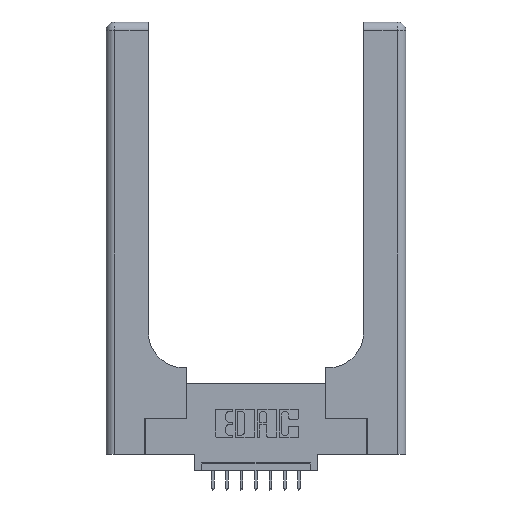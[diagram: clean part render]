
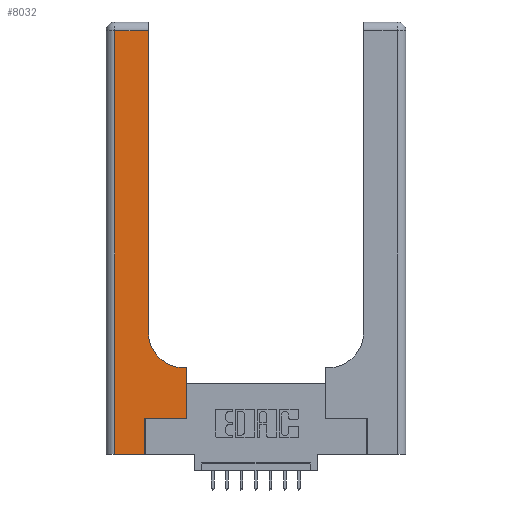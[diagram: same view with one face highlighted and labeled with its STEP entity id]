
A CAD part, top view. The second image highlights one B-rep face of the part: STEP entity #8032.
In plain terms, the highlighted planar face has unit normal (0, 0, 1).
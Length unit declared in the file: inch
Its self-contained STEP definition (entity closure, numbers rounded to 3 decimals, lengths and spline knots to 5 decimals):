
#13 = CARTESIAN_POINT ( 'NONE',  ( 0.5415, 0.85, 0.37 ) ) ;
#379 = EDGE_CURVE ( 'NONE', #5066, #6517, #4781, .T. ) ;
#677 = VERTEX_POINT ( 'NONE', #11821 ) ;
#979 = VERTEX_POINT ( 'NONE', #9960 ) ;
#1212 = DIRECTION ( 'NONE',  ( -1., 0., 0. ) ) ;
#1275 = CARTESIAN_POINT ( 'NONE',  ( 0.5585, 0.6, 0.37 ) ) ;
#1513 = EDGE_CURVE ( 'NONE', #6517, #6778, #9092, .T. ) ;
#1852 = ORIENTED_EDGE ( 'NONE', *, *, #12530, .T. ) ;
#1937 = ORIENTED_EDGE ( 'NONE', *, *, #12437, .T. ) ;
#2264 = CARTESIAN_POINT ( 'NONE',  ( 0.2915, 2.94, 0.37 ) ) ;
#2290 = CARTESIAN_POINT ( 'NONE',  ( 0., 0., 0.37 ) ) ;
#2547 = EDGE_CURVE ( 'NONE', #677, #979, #7490, .T. ) ;
#2869 = ORIENTED_EDGE ( 'NONE', *, *, #7339, .T. ) ;
#3173 = CARTESIAN_POINT ( 'NONE',  ( 0., 3., 0.37 ) ) ;
#3446 = VERTEX_POINT ( 'NONE', #1275 ) ;
#3623 = VERTEX_POINT ( 'NONE', #10131 ) ;
#4225 = CARTESIAN_POINT ( 'NONE',  ( 0.269, 0., 0.37 ) ) ;
#4233 = EDGE_CURVE ( 'NONE', #14775, #5066, #8551, .T. ) ;
#4272 = LINE ( 'NONE', #11412, #5386 ) ;
#4508 = DIRECTION ( 'NONE',  ( 0., 1., 0. ) ) ;
#4589 = AXIS2_PLACEMENT_3D ( 'NONE', #3173, #8083, #10240 ) ;
#4781 = LINE ( 'NONE', #5859, #12461 ) ;
#5066 = VERTEX_POINT ( 'NONE', #2264 ) ;
#5340 = VECTOR ( 'NONE', #1212, 39.37008 ) ;
#5386 = VECTOR ( 'NONE', #4508, 39.37008 ) ;
#5387 = DIRECTION ( 'NONE',  ( 0., 1., 0. ) ) ;
#5513 = ORIENTED_EDGE ( 'NONE', *, *, #11444, .T. ) ;
#5607 = CARTESIAN_POINT ( 'NONE',  ( 0.2915, 0.85, 0.37 ) ) ;
#5635 = DIRECTION ( 'NONE',  ( 1., 0., 0. ) ) ;
#5810 = CIRCLE ( 'NONE', #8811, 0.25 ) ;
#5859 = CARTESIAN_POINT ( 'NONE',  ( 0., 2.94, 0.37 ) ) ;
#6038 = CARTESIAN_POINT ( 'NONE',  ( 0.2915, 0.6, 0.37 ) ) ;
#6109 = VECTOR ( 'NONE', #10857, 39.37008 ) ;
#6148 = VERTEX_POINT ( 'NONE', #12683 ) ;
#6517 = VERTEX_POINT ( 'NONE', #12822 ) ;
#6778 = VERTEX_POINT ( 'NONE', #12315 ) ;
#6878 = DIRECTION ( 'NONE',  ( 0., 0., -1. ) ) ;
#7144 = DIRECTION ( 'NONE',  ( 0., 1., 0. ) ) ;
#7339 = EDGE_CURVE ( 'NONE', #3623, #14775, #5810, .T. ) ;
#7490 = LINE ( 'NONE', #4225, #11481 ) ;
#8032 = ADVANCED_FACE ( 'NONE', ( #15076 ), #13963, .F. ) ;
#8083 = DIRECTION ( 'NONE',  ( 0., 0., -1. ) ) ;
#8469 = ORIENTED_EDGE ( 'NONE', *, *, #1513, .T. ) ;
#8551 = LINE ( 'NONE', #12104, #10769 ) ;
#8811 = AXIS2_PLACEMENT_3D ( 'NONE', #13, #6878, #5635 ) ;
#9092 = LINE ( 'NONE', #10094, #9782 ) ;
#9184 = CARTESIAN_POINT ( 'NONE',  ( 0.269, 0.25, 0.37 ) ) ;
#9638 = LINE ( 'NONE', #2290, #6109 ) ;
#9782 = VECTOR ( 'NONE', #10015, 39.37008 ) ;
#9960 = CARTESIAN_POINT ( 'NONE',  ( 0.269, 0.25, 0.37 ) ) ;
#10015 = DIRECTION ( 'NONE',  ( 0., -1., 0. ) ) ;
#10094 = CARTESIAN_POINT ( 'NONE',  ( 0.06, 3., 0.37 ) ) ;
#10098 = VECTOR ( 'NONE', #11482, 39.37008 ) ;
#10131 = CARTESIAN_POINT ( 'NONE',  ( 0.5415, 0.6, 0.37 ) ) ;
#10240 = DIRECTION ( 'NONE',  ( -1., 0., 0. ) ) ;
#10252 = EDGE_CURVE ( 'NONE', #3446, #3623, #13101, .T. ) ;
#10515 = DIRECTION ( 'NONE',  ( -1., 0., 0. ) ) ;
#10750 = ORIENTED_EDGE ( 'NONE', *, *, #379, .T. ) ;
#10769 = VECTOR ( 'NONE', #7144, 39.37008 ) ;
#10857 = DIRECTION ( 'NONE',  ( 1., 0., 0. ) ) ;
#10858 = ORIENTED_EDGE ( 'NONE', *, *, #10252, .T. ) ;
#11412 = CARTESIAN_POINT ( 'NONE',  ( 0.5585, 0.25, 0.37 ) ) ;
#11444 = EDGE_CURVE ( 'NONE', #6778, #677, #9638, .T. ) ;
#11481 = VECTOR ( 'NONE', #5387, 39.37008 ) ;
#11482 = DIRECTION ( 'NONE',  ( 1., 0., 0. ) ) ;
#11821 = CARTESIAN_POINT ( 'NONE',  ( 0.269, 0., 0.37 ) ) ;
#11853 = ORIENTED_EDGE ( 'NONE', *, *, #4233, .T. ) ;
#12104 = CARTESIAN_POINT ( 'NONE',  ( 0.2915, 3., 0.37 ) ) ;
#12315 = CARTESIAN_POINT ( 'NONE',  ( 0.06, 0., 0.37 ) ) ;
#12437 = EDGE_CURVE ( 'NONE', #6148, #3446, #4272, .T. ) ;
#12461 = VECTOR ( 'NONE', #10515, 39.37008 ) ;
#12530 = EDGE_CURVE ( 'NONE', #979, #6148, #13970, .T. ) ;
#12683 = CARTESIAN_POINT ( 'NONE',  ( 0.5585, 0.25, 0.37 ) ) ;
#12822 = CARTESIAN_POINT ( 'NONE',  ( 0.06, 2.94, 0.37 ) ) ;
#13101 = LINE ( 'NONE', #6038, #5340 ) ;
#13883 = EDGE_LOOP ( 'NONE', ( #11853, #10750, #8469, #5513, #14255, #1852, #1937, #10858, #2869 ) ) ;
#13963 = PLANE ( 'NONE',  #4589 ) ;
#13970 = LINE ( 'NONE', #9184, #10098 ) ;
#14255 = ORIENTED_EDGE ( 'NONE', *, *, #2547, .T. ) ;
#14775 = VERTEX_POINT ( 'NONE', #5607 ) ;
#15076 = FACE_OUTER_BOUND ( 'NONE', #13883, .T. ) ;
